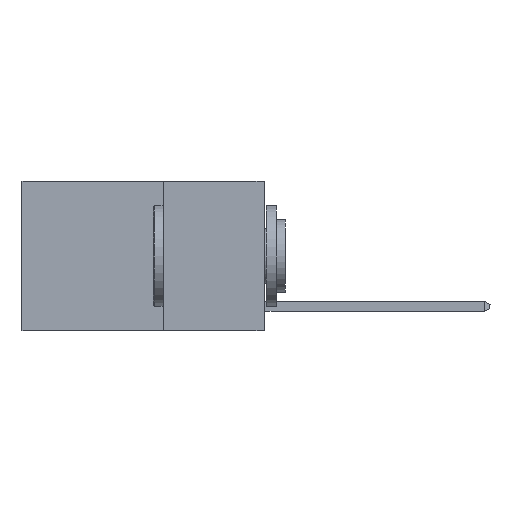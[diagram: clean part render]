
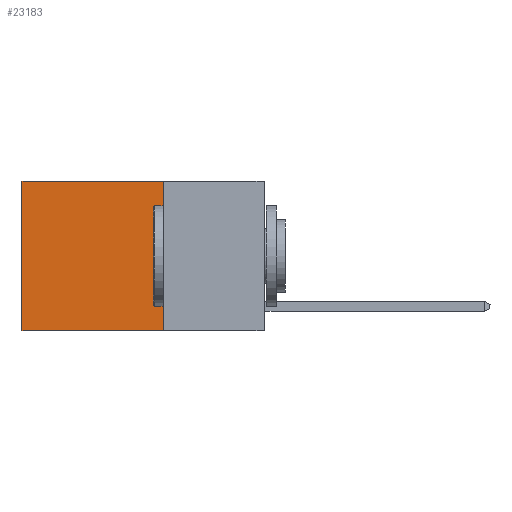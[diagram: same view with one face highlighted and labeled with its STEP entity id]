
A CAD part, left-side view. The second image highlights one B-rep face of the part: STEP entity #23183.
In plain terms, the highlighted planar face has unit normal (-1, 0, 0).
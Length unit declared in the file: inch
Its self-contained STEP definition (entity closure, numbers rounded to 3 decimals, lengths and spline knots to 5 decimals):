
#1004 = DIRECTION ( 'NONE',  ( 0., 0., -1. ) ) ;
#1766 = EDGE_LOOP ( 'NONE', ( #12883, #7771, #4846, #18689 ) ) ;
#2395 = VECTOR ( 'NONE', #17328, 39.37008 ) ;
#2469 = VERTEX_POINT ( 'NONE', #4994 ) ;
#3137 = CARTESIAN_POINT ( 'NONE',  ( 0.2625, 0.25, 0. ) ) ;
#4797 = DIRECTION ( 'NONE',  ( 1., 0., 0. ) ) ;
#4846 = ORIENTED_EDGE ( 'NONE', *, *, #18670, .F. ) ;
#4994 = CARTESIAN_POINT ( 'NONE',  ( 0.2625, 0.6, -0.37 ) ) ;
#6138 = CARTESIAN_POINT ( 'NONE',  ( 0.2625, 0.6, 0. ) ) ;
#6591 = FACE_OUTER_BOUND ( 'NONE', #1766, .T. ) ;
#7771 = ORIENTED_EDGE ( 'NONE', *, *, #18228, .F. ) ;
#7856 = VECTOR ( 'NONE', #14022, 39.37008 ) ;
#7969 = DIRECTION ( 'NONE',  ( 0., 0., -1. ) ) ;
#8213 = VECTOR ( 'NONE', #7969, 39.37008 ) ;
#8294 = CARTESIAN_POINT ( 'NONE',  ( 0.2625, 0.25, -0.37 ) ) ;
#8414 = DIRECTION ( 'NONE',  ( 0., 0., -1. ) ) ;
#8493 = EDGE_CURVE ( 'NONE', #17327, #13430, #10430, .T. ) ;
#8657 = CARTESIAN_POINT ( 'NONE',  ( 0.2625, 0.25, 0. ) ) ;
#9098 = CARTESIAN_POINT ( 'NONE',  ( 0.2625, 0.25, -0.37 ) ) ;
#10232 = CARTESIAN_POINT ( 'NONE',  ( 0.2625, 0.25, 0. ) ) ;
#10363 = LINE ( 'NONE', #8657, #14157 ) ;
#10430 = LINE ( 'NONE', #3137, #7856 ) ;
#10685 = VERTEX_POINT ( 'NONE', #8294 ) ;
#12883 = ORIENTED_EDGE ( 'NONE', *, *, #20186, .T. ) ;
#13430 = VERTEX_POINT ( 'NONE', #24162 ) ;
#13451 = AXIS2_PLACEMENT_3D ( 'NONE', #10232, #4797, #1004 ) ;
#14022 = DIRECTION ( 'NONE',  ( 0., 1., 0. ) ) ;
#14157 = VECTOR ( 'NONE', #8414, 39.37008 ) ;
#15367 = LINE ( 'NONE', #6138, #8213 ) ;
#17327 = VERTEX_POINT ( 'NONE', #19204 ) ;
#17328 = DIRECTION ( 'NONE',  ( 0., 1., 0. ) ) ;
#17784 = PLANE ( 'NONE',  #13451 ) ;
#18228 = EDGE_CURVE ( 'NONE', #10685, #2469, #23133, .T. ) ;
#18670 = EDGE_CURVE ( 'NONE', #17327, #10685, #10363, .T. ) ;
#18689 = ORIENTED_EDGE ( 'NONE', *, *, #8493, .T. ) ;
#19204 = CARTESIAN_POINT ( 'NONE',  ( 0.2625, 0.25, 0. ) ) ;
#20186 = EDGE_CURVE ( 'NONE', #13430, #2469, #15367, .T. ) ;
#23133 = LINE ( 'NONE', #9098, #2395 ) ;
#23183 = ADVANCED_FACE ( 'NONE', ( #6591 ), #17784, .F. ) ;
#24162 = CARTESIAN_POINT ( 'NONE',  ( 0.2625, 0.6, 0. ) ) ;
